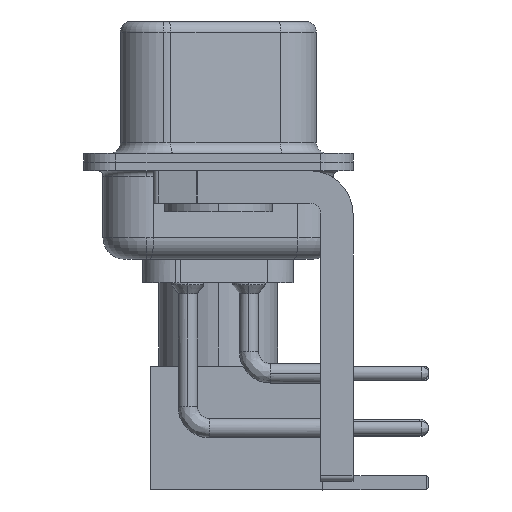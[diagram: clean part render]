
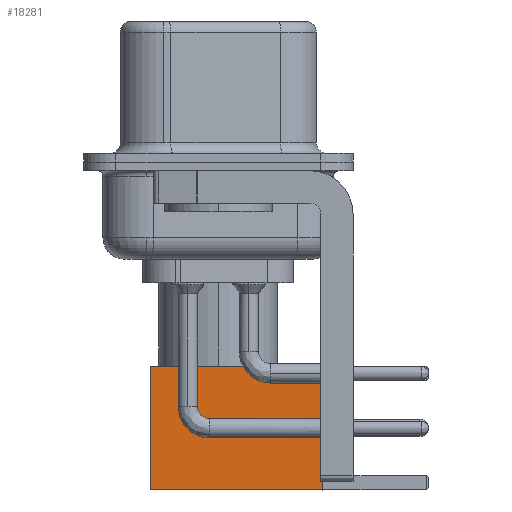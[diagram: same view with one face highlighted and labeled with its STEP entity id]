
A CAD part, left-side view. The second image highlights one B-rep face of the part: STEP entity #18281.
In plain terms, the highlighted face is planar.
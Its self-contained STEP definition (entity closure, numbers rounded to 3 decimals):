
#93 = VERTEX_POINT ( 'NONE', #4038 ) ;
#153 = VECTOR ( 'NONE', #9413, 1000. ) ;
#887 = CARTESIAN_POINT ( 'NONE',  ( 2.875, 2.875, 8. ) ) ;
#2328 = EDGE_CURVE ( 'NONE', #16856, #10731, #29986, .T. ) ;
#4038 = CARTESIAN_POINT ( 'NONE',  ( 2.875, 2.875, 0. ) ) ;
#6540 = DIRECTION ( 'NONE',  ( 0., 0., 1. ) ) ;
#8119 = DIRECTION ( 'NONE',  ( 0., 0., -1. ) ) ;
#8791 = DIRECTION ( 'NONE',  ( -1., 0., 0. ) ) ;
#9172 = PLANE ( 'NONE',  #15245 ) ;
#9413 = DIRECTION ( 'NONE',  ( -1., 0., 0. ) ) ;
#9821 = VECTOR ( 'NONE', #8119, 1000. ) ;
#9981 = VECTOR ( 'NONE', #8791, 1000. ) ;
#10731 = VERTEX_POINT ( 'NONE', #29475 ) ;
#12110 = CARTESIAN_POINT ( 'NONE',  ( -2.875, 2.875, 0. ) ) ;
#12470 = LINE ( 'NONE', #22508, #9821 ) ;
#14607 = VECTOR ( 'NONE', #26031, 1000. ) ;
#15245 = AXIS2_PLACEMENT_3D ( 'NONE', #20641, #15693, #6540 ) ;
#15374 = VERTEX_POINT ( 'NONE', #20672 ) ;
#15693 = DIRECTION ( 'NONE',  ( 0., 1., 0. ) ) ;
#16826 = ORIENTED_EDGE ( 'NONE', *, *, #22815, .F. ) ;
#16856 = VERTEX_POINT ( 'NONE', #887 ) ;
#18281 = ADVANCED_FACE ( 'NONE', ( #23263 ), #9172, .T. ) ;
#18965 = CARTESIAN_POINT ( 'NONE',  ( 0., 2.875, 8. ) ) ;
#19056 = EDGE_CURVE ( 'NONE', #16856, #93, #12470, .T. ) ;
#19763 = EDGE_LOOP ( 'NONE', ( #28273, #24689, #16826, #20903 ) ) ;
#20641 = CARTESIAN_POINT ( 'NONE',  ( 2.875, 2.875, 0. ) ) ;
#20672 = CARTESIAN_POINT ( 'NONE',  ( -2.875, 2.875, 0. ) ) ;
#20826 = EDGE_CURVE ( 'NONE', #93, #15374, #28123, .T. ) ;
#20903 = ORIENTED_EDGE ( 'NONE', *, *, #2328, .F. ) ;
#22508 = CARTESIAN_POINT ( 'NONE',  ( 2.875, 2.875, 0. ) ) ;
#22815 = EDGE_CURVE ( 'NONE', #10731, #15374, #23570, .T. ) ;
#23263 = FACE_OUTER_BOUND ( 'NONE', #19763, .T. ) ;
#23570 = LINE ( 'NONE', #12110, #14607 ) ;
#24689 = ORIENTED_EDGE ( 'NONE', *, *, #20826, .T. ) ;
#25809 = CARTESIAN_POINT ( 'NONE',  ( 0., 2.875, 0. ) ) ;
#26031 = DIRECTION ( 'NONE',  ( 0., 0., -1. ) ) ;
#28123 = LINE ( 'NONE', #25809, #153 ) ;
#28273 = ORIENTED_EDGE ( 'NONE', *, *, #19056, .T. ) ;
#29475 = CARTESIAN_POINT ( 'NONE',  ( -2.875, 2.875, 8. ) ) ;
#29986 = LINE ( 'NONE', #18965, #9981 ) ;
